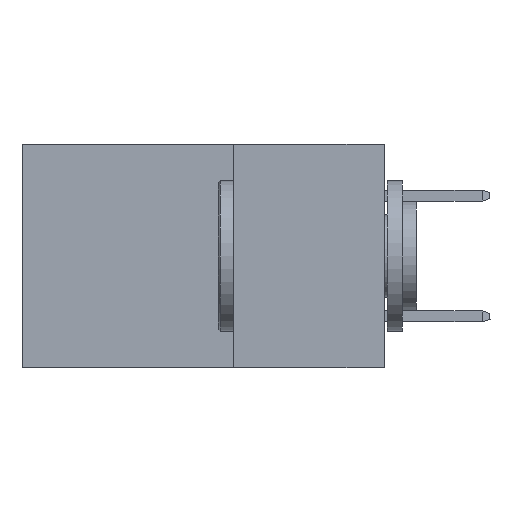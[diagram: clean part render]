
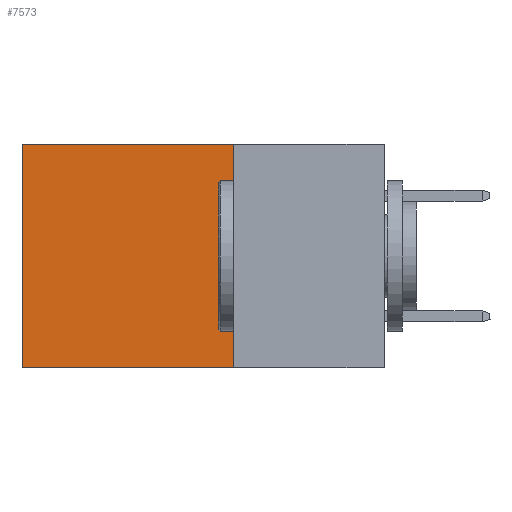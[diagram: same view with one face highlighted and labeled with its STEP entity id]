
A CAD part, left-side view. The second image highlights one B-rep face of the part: STEP entity #7573.
In plain terms, the highlighted planar face has unit normal (-1, 0, 0).
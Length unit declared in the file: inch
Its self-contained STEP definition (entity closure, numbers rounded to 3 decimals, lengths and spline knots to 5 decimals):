
#1038 = CARTESIAN_POINT ( 'NONE',  ( 0.2615, 0.6, 0. ) ) ;
#1053 = DIRECTION ( 'NONE',  ( 0., 1., 0. ) ) ;
#1119 = CARTESIAN_POINT ( 'NONE',  ( 0.2615, 0.25, 0. ) ) ;
#2108 = DIRECTION ( 'NONE',  ( 1., 0., 0. ) ) ;
#2415 = ORIENTED_EDGE ( 'NONE', *, *, #13453, .F. ) ;
#3336 = VERTEX_POINT ( 'NONE', #16344 ) ;
#3377 = CARTESIAN_POINT ( 'NONE',  ( 0.2615, 0.25, -0.37 ) ) ;
#4463 = LINE ( 'NONE', #1119, #16191 ) ;
#4926 = DIRECTION ( 'NONE',  ( 0., 0., -1. ) ) ;
#5176 = PLANE ( 'NONE',  #11831 ) ;
#5522 = DIRECTION ( 'NONE',  ( 0., 1., 0. ) ) ;
#6100 = EDGE_CURVE ( 'NONE', #14723, #7806, #4463, .T. ) ;
#6390 = VECTOR ( 'NONE', #13403, 39.37008 ) ;
#7573 = ADVANCED_FACE ( 'NONE', ( #20127 ), #5176, .F. ) ;
#7806 = VERTEX_POINT ( 'NONE', #1038 ) ;
#8536 = CARTESIAN_POINT ( 'NONE',  ( 0.2615, 0.25, -0.37 ) ) ;
#9436 = ORIENTED_EDGE ( 'NONE', *, *, #6100, .T. ) ;
#9579 = CARTESIAN_POINT ( 'NONE',  ( 0.2615, 0.25, 0. ) ) ;
#10607 = VECTOR ( 'NONE', #5522, 39.37008 ) ;
#10708 = LINE ( 'NONE', #18094, #6390 ) ;
#10863 = EDGE_LOOP ( 'NONE', ( #17538, #12004, #2415, #9436 ) ) ;
#11008 = VERTEX_POINT ( 'NONE', #8536 ) ;
#11673 = CARTESIAN_POINT ( 'NONE',  ( 0.2615, 0.25, -0.37 ) ) ;
#11831 = AXIS2_PLACEMENT_3D ( 'NONE', #11673, #2108, #13262 ) ;
#12004 = ORIENTED_EDGE ( 'NONE', *, *, #20221, .F. ) ;
#13262 = DIRECTION ( 'NONE',  ( 0., 0., -1. ) ) ;
#13403 = DIRECTION ( 'NONE',  ( 0., 0., -1. ) ) ;
#13453 = EDGE_CURVE ( 'NONE', #14723, #11008, #20270, .T. ) ;
#13563 = CARTESIAN_POINT ( 'NONE',  ( 0.2615, 0.25, -0.37 ) ) ;
#14723 = VERTEX_POINT ( 'NONE', #9579 ) ;
#14835 = LINE ( 'NONE', #13563, #10607 ) ;
#16191 = VECTOR ( 'NONE', #1053, 39.37008 ) ;
#16344 = CARTESIAN_POINT ( 'NONE',  ( 0.2615, 0.6, -0.37 ) ) ;
#17538 = ORIENTED_EDGE ( 'NONE', *, *, #18028, .T. ) ;
#18028 = EDGE_CURVE ( 'NONE', #7806, #3336, #10708, .T. ) ;
#18094 = CARTESIAN_POINT ( 'NONE',  ( 0.2615, 0.6, -0.37 ) ) ;
#19778 = VECTOR ( 'NONE', #4926, 39.37008 ) ;
#20127 = FACE_OUTER_BOUND ( 'NONE', #10863, .T. ) ;
#20221 = EDGE_CURVE ( 'NONE', #11008, #3336, #14835, .T. ) ;
#20270 = LINE ( 'NONE', #3377, #19778 ) ;
